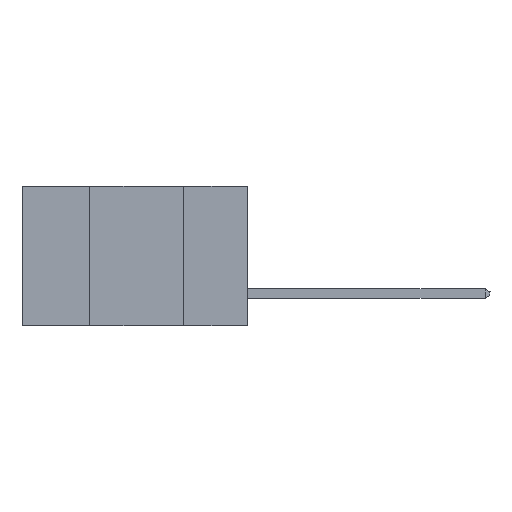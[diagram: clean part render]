
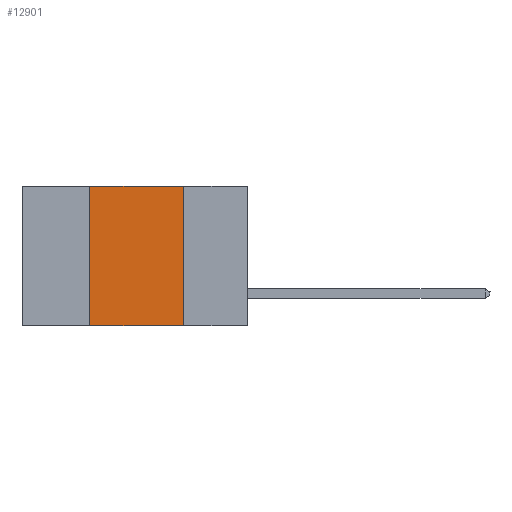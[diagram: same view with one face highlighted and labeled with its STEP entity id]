
A CAD part, left-side view. The second image highlights one B-rep face of the part: STEP entity #12901.
In plain terms, the highlighted planar face has unit normal (-1, 0, 0).
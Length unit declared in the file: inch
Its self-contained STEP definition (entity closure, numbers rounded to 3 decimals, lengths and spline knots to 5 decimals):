
#683 = ORIENTED_EDGE ( 'NONE', *, *, #15449, .F. ) ;
#1933 = LINE ( 'NONE', #16194, #11575 ) ;
#1999 = DIRECTION ( 'NONE',  ( 0., 0., -1. ) ) ;
#2077 = DIRECTION ( 'NONE',  ( 0., 0., -1. ) ) ;
#3036 = EDGE_LOOP ( 'NONE', ( #683, #15165, #5984, #8467 ) ) ;
#3298 = LINE ( 'NONE', #16957, #5595 ) ;
#3445 = LINE ( 'NONE', #5074, #10142 ) ;
#3930 = AXIS2_PLACEMENT_3D ( 'NONE', #4637, #17310, #1999 ) ;
#3931 = CARTESIAN_POINT ( 'NONE',  ( 0., 0.42, 0. ) ) ;
#4055 = CARTESIAN_POINT ( 'NONE',  ( 0., 0.42, -0.37 ) ) ;
#4199 = VERTEX_POINT ( 'NONE', #9878 ) ;
#4374 = DIRECTION ( 'NONE',  ( 0., -1., 0. ) ) ;
#4561 = VECTOR ( 'NONE', #8280, 39.37008 ) ;
#4637 = CARTESIAN_POINT ( 'NONE',  ( 0., 0.6, 0. ) ) ;
#5074 = CARTESIAN_POINT ( 'NONE',  ( 0., 0.17, -0.37 ) ) ;
#5359 = EDGE_CURVE ( 'NONE', #11437, #4199, #12494, .T. ) ;
#5595 = VECTOR ( 'NONE', #4374, 39.37008 ) ;
#5814 = EDGE_CURVE ( 'NONE', #9457, #13551, #3298, .T. ) ;
#5984 = ORIENTED_EDGE ( 'NONE', *, *, #11523, .F. ) ;
#6967 = CARTESIAN_POINT ( 'NONE',  ( 0., 0.17, -0.37 ) ) ;
#8280 = DIRECTION ( 'NONE',  ( 0., -1., 0. ) ) ;
#8467 = ORIENTED_EDGE ( 'NONE', *, *, #5814, .T. ) ;
#9457 = VERTEX_POINT ( 'NONE', #4055 ) ;
#9878 = CARTESIAN_POINT ( 'NONE',  ( 0., 0.17, 0. ) ) ;
#10142 = VECTOR ( 'NONE', #2077, 39.37008 ) ;
#10275 = DIRECTION ( 'NONE',  ( 0., 0., 1. ) ) ;
#11437 = VERTEX_POINT ( 'NONE', #3931 ) ;
#11518 = FACE_OUTER_BOUND ( 'NONE', #3036, .T. ) ;
#11523 = EDGE_CURVE ( 'NONE', #9457, #11437, #1933, .T. ) ;
#11575 = VECTOR ( 'NONE', #10275, 39.37008 ) ;
#12494 = LINE ( 'NONE', #18107, #4561 ) ;
#12901 = ADVANCED_FACE ( 'NONE', ( #11518 ), #14459, .F. ) ;
#13551 = VERTEX_POINT ( 'NONE', #6967 ) ;
#14459 = PLANE ( 'NONE',  #3930 ) ;
#15165 = ORIENTED_EDGE ( 'NONE', *, *, #5359, .F. ) ;
#15449 = EDGE_CURVE ( 'NONE', #4199, #13551, #3445, .T. ) ;
#16194 = CARTESIAN_POINT ( 'NONE',  ( 0., 0.42, -0.37 ) ) ;
#16957 = CARTESIAN_POINT ( 'NONE',  ( 0., 0.6, -0.37 ) ) ;
#17310 = DIRECTION ( 'NONE',  ( 1., 0., 0. ) ) ;
#18107 = CARTESIAN_POINT ( 'NONE',  ( 0., 0.6, 0. ) ) ;
